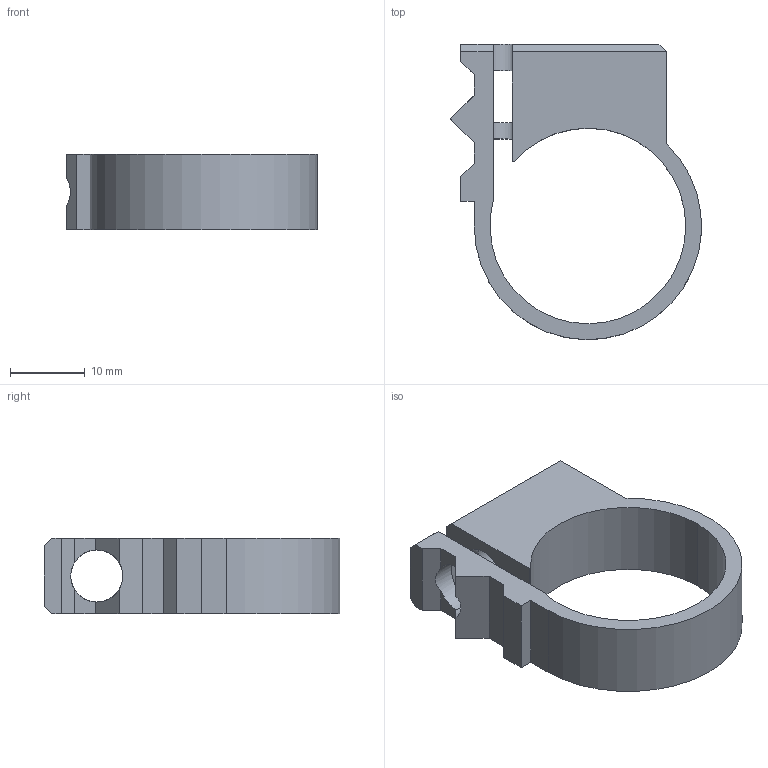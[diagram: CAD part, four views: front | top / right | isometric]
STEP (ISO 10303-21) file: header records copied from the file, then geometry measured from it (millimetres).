
FILE_DESCRIPTION (( 'STEP AP203' ), '1' );
FILE_NAME ('AF-WF-MI-PRT-003-STL.STEP', '2020-07-21T23:45:06', ( '' ), ( '' ), 'SwSTEP 2.0', 'SolidWorks 2018', '' );
FILE_SCHEMA (( 'CONFIG_CONTROL_DESIGN' ));
Length unit declared in the file: inch
Products named in the file (1): AF-WF-MI-PRT-003-STL
Bounding box: 33.63 x 39.6 x 10.16 mm (x, y, z)
Volume: 3767 mm3; surface area: 3784.1 mm2
Topology: 1 solids, 1 shells, 41 faces, 118 edges, 78 vertices
Faces by surface type: plane 29, cylinder 12
Entity records: 1489 total; most frequent: CARTESIAN_POINT 322, ORIENTED_EDGE 236, DIRECTION 218, EDGE_CURVE 118, VECTOR 86, LINE 86, VERTEX_POINT 78, AXIS2_PLACEMENT_3D 66
